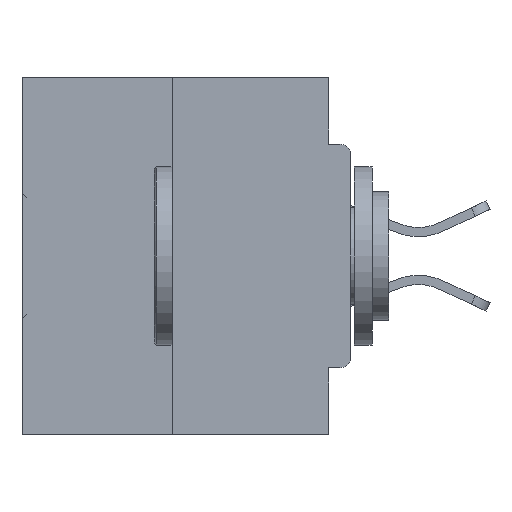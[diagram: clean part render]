
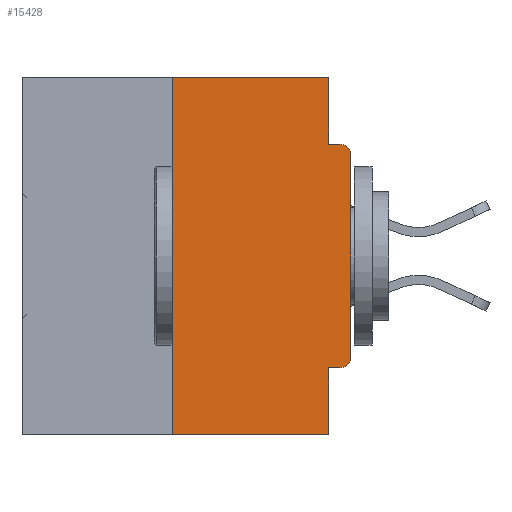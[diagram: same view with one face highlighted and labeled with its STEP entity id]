
A CAD part, left-side view. The second image highlights one B-rep face of the part: STEP entity #15428.
In plain terms, the highlighted planar face has unit normal (-1, 0, 0).
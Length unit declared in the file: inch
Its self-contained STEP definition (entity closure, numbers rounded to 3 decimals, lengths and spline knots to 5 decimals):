
#354 = LINE ( 'NONE', #41308, #8103 ) ;
#414 = VERTEX_POINT ( 'NONE', #41234 ) ;
#450 = ORIENTED_EDGE ( 'NONE', *, *, #25473, .F. ) ;
#731 = DIRECTION ( 'NONE',  ( 0., -1., 0. ) ) ;
#2478 = EDGE_CURVE ( 'NONE', #44881, #40959, #9907, .T. ) ;
#3312 = DIRECTION ( 'NONE',  ( -1., 0., 0. ) ) ;
#3830 = PLANE ( 'NONE',  #33964 ) ;
#4809 = CIRCLE ( 'NONE', #32314, 0.015 ) ;
#5221 = CARTESIAN_POINT ( 'NONE',  ( 0., 0., -0.4065 ) ) ;
#6780 = EDGE_CURVE ( 'NONE', #414, #28340, #15576, .T. ) ;
#7376 = DIRECTION ( 'NONE',  ( 0., 0., -1. ) ) ;
#8022 = VERTEX_POINT ( 'NONE', #37242 ) ;
#8103 = VECTOR ( 'NONE', #41159, 39.37008 ) ;
#8664 = CARTESIAN_POINT ( 'NONE',  ( 0., 0.46, 0. ) ) ;
#8818 = VECTOR ( 'NONE', #43932, 39.37008 ) ;
#9907 = LINE ( 'NONE', #8664, #8818 ) ;
#10180 = EDGE_CURVE ( 'NONE', #8022, #38962, #16967, .T. ) ;
#10738 = CARTESIAN_POINT ( 'NONE',  ( 0., 0.031, -0.4065 ) ) ;
#10819 = ORIENTED_EDGE ( 'NONE', *, *, #23618, .F. ) ;
#11187 = CARTESIAN_POINT ( 'NONE',  ( 0., 0.015, -0.1085 ) ) ;
#13249 = VECTOR ( 'NONE', #7376, 39.37008 ) ;
#13538 = CARTESIAN_POINT ( 'NONE',  ( 0., 0., -0.3915 ) ) ;
#13738 = ORIENTED_EDGE ( 'NONE', *, *, #22294, .T. ) ;
#13923 = CARTESIAN_POINT ( 'NONE',  ( 0., 0.25, 0. ) ) ;
#14095 = EDGE_CURVE ( 'NONE', #40875, #44881, #20575, .T. ) ;
#14112 = DIRECTION ( 'NONE',  ( 0., 0., -1. ) ) ;
#14296 = EDGE_CURVE ( 'NONE', #28340, #35418, #36140, .T. ) ;
#15428 = ADVANCED_FACE ( 'NONE', ( #29672 ), #3830, .F. ) ;
#15576 = CIRCLE ( 'NONE', #17308, 0.015 ) ;
#16967 = LINE ( 'NONE', #39564, #25285 ) ;
#17308 = AXIS2_PLACEMENT_3D ( 'NONE', #25006, #3312, #14112 ) ;
#18011 = VECTOR ( 'NONE', #29439, 39.37008 ) ;
#19246 = CARTESIAN_POINT ( 'NONE',  ( 0., 0.46, -0.5 ) ) ;
#19515 = VECTOR ( 'NONE', #31011, 39.37008 ) ;
#20262 = ORIENTED_EDGE ( 'NONE', *, *, #2478, .F. ) ;
#20473 = ORIENTED_EDGE ( 'NONE', *, *, #20695, .T. ) ;
#20575 = LINE ( 'NONE', #27099, #28845 ) ;
#20695 = EDGE_CURVE ( 'NONE', #35418, #38962, #4809, .T. ) ;
#21393 = DIRECTION ( 'NONE',  ( 1., 0., 0. ) ) ;
#21552 = DIRECTION ( 'NONE',  ( 0., 0., -1. ) ) ;
#21772 = DIRECTION ( 'NONE',  ( -1., 0., 0. ) ) ;
#22294 = EDGE_CURVE ( 'NONE', #40875, #42109, #36875, .T. ) ;
#22921 = ORIENTED_EDGE ( 'NONE', *, *, #10180, .F. ) ;
#23333 = CARTESIAN_POINT ( 'NONE',  ( 0., 0.25, -0.5 ) ) ;
#23618 = EDGE_CURVE ( 'NONE', #414, #25424, #33959, .T. ) ;
#24440 = CARTESIAN_POINT ( 'NONE',  ( 0., 0.031, -0.5 ) ) ;
#24788 = CARTESIAN_POINT ( 'NONE',  ( 0., 0.46, 0. ) ) ;
#25006 = CARTESIAN_POINT ( 'NONE',  ( 0., 0.015, -0.3915 ) ) ;
#25285 = VECTOR ( 'NONE', #731, 39.37008 ) ;
#25424 = VERTEX_POINT ( 'NONE', #10738 ) ;
#25473 = EDGE_CURVE ( 'NONE', #25424, #42109, #32123, .T. ) ;
#27099 = CARTESIAN_POINT ( 'NONE',  ( 0., 0.25, 0. ) ) ;
#28176 = EDGE_LOOP ( 'NONE', ( #20262, #37613, #13738, #450, #10819, #33699, #31987, #20473, #22921, #42422 ) ) ;
#28340 = VERTEX_POINT ( 'NONE', #13538 ) ;
#28845 = VECTOR ( 'NONE', #37779, 39.37008 ) ;
#29173 = DIRECTION ( 'NONE',  ( 0., 0., -1. ) ) ;
#29439 = DIRECTION ( 'NONE',  ( 0., -1., 0. ) ) ;
#29672 = FACE_OUTER_BOUND ( 'NONE', #28176, .T. ) ;
#30027 = DIRECTION ( 'NONE',  ( 0., 1., 0. ) ) ;
#31011 = DIRECTION ( 'NONE',  ( 0., 0., 1. ) ) ;
#31987 = ORIENTED_EDGE ( 'NONE', *, *, #14296, .T. ) ;
#32123 = LINE ( 'NONE', #24440, #13249 ) ;
#32288 = VECTOR ( 'NONE', #30027, 39.37008 ) ;
#32314 = AXIS2_PLACEMENT_3D ( 'NONE', #11187, #21772, #29173 ) ;
#33699 = ORIENTED_EDGE ( 'NONE', *, *, #6780, .T. ) ;
#33959 = LINE ( 'NONE', #5221, #32288 ) ;
#33964 = AXIS2_PLACEMENT_3D ( 'NONE', #24788, #21393, #21552 ) ;
#34265 = CARTESIAN_POINT ( 'NONE',  ( 0., 0., 0. ) ) ;
#34442 = CARTESIAN_POINT ( 'NONE',  ( 0., 0.031, 0. ) ) ;
#34694 = EDGE_CURVE ( 'NONE', #40959, #8022, #354, .T. ) ;
#35418 = VERTEX_POINT ( 'NONE', #37989 ) ;
#36140 = LINE ( 'NONE', #34265, #19515 ) ;
#36875 = LINE ( 'NONE', #19246, #18011 ) ;
#37242 = CARTESIAN_POINT ( 'NONE',  ( 0., 0.031, -0.0935 ) ) ;
#37613 = ORIENTED_EDGE ( 'NONE', *, *, #14095, .F. ) ;
#37779 = DIRECTION ( 'NONE',  ( 0., 0., 1. ) ) ;
#37989 = CARTESIAN_POINT ( 'NONE',  ( 0., 0., -0.1085 ) ) ;
#38962 = VERTEX_POINT ( 'NONE', #43152 ) ;
#39564 = CARTESIAN_POINT ( 'NONE',  ( 0., 0., -0.0935 ) ) ;
#40875 = VERTEX_POINT ( 'NONE', #23333 ) ;
#40959 = VERTEX_POINT ( 'NONE', #34442 ) ;
#41159 = DIRECTION ( 'NONE',  ( 0., 0., -1. ) ) ;
#41234 = CARTESIAN_POINT ( 'NONE',  ( 0., 0.015, -0.4065 ) ) ;
#41308 = CARTESIAN_POINT ( 'NONE',  ( 0., 0.031, 0. ) ) ;
#42109 = VERTEX_POINT ( 'NONE', #43897 ) ;
#42422 = ORIENTED_EDGE ( 'NONE', *, *, #34694, .F. ) ;
#43152 = CARTESIAN_POINT ( 'NONE',  ( 0., 0.015, -0.0935 ) ) ;
#43897 = CARTESIAN_POINT ( 'NONE',  ( 0., 0.031, -0.5 ) ) ;
#43932 = DIRECTION ( 'NONE',  ( 0., -1., 0. ) ) ;
#44881 = VERTEX_POINT ( 'NONE', #13923 ) ;
